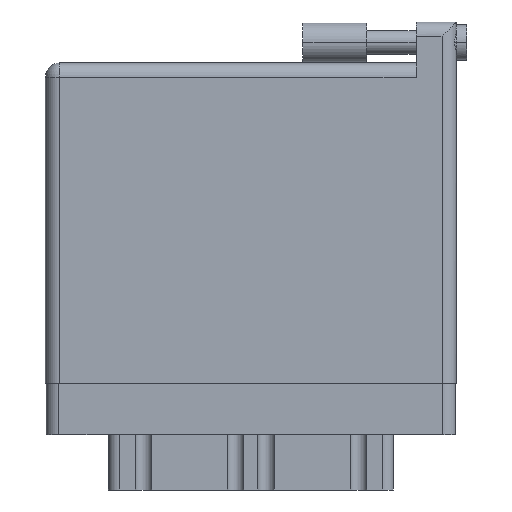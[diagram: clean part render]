
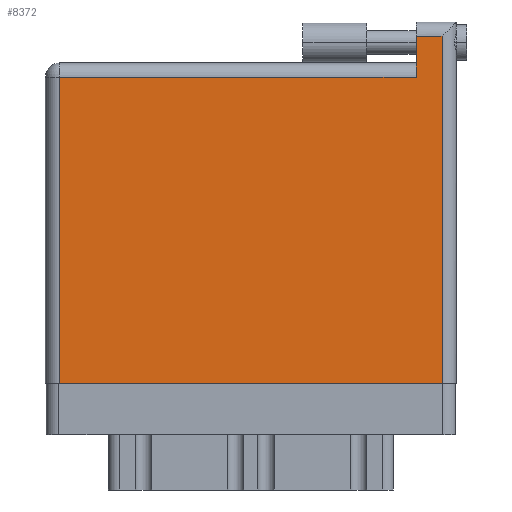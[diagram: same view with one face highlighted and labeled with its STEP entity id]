
A CAD part, front view. The second image highlights one B-rep face of the part: STEP entity #8372.
In plain terms, the highlighted face is planar.
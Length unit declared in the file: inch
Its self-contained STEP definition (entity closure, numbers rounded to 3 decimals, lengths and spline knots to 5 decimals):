
#135 = CARTESIAN_POINT ( 'NONE',  ( 0.07, 0., 0. ) ) ;
#1037 = CARTESIAN_POINT ( 'NONE',  ( 0., 1.696, 0. ) ) ;
#4168 = ORIENTED_EDGE ( 'NONE', *, *, #9324, .T. ) ;
#5502 = CARTESIAN_POINT ( 'NONE',  ( 0., 0., 0. ) ) ;
#5734 = DIRECTION ( 'NONE',  ( -1., 0., 0. ) ) ;
#6928 = LINE ( 'NONE', #24850, #19452 ) ;
#8372 = ADVANCED_FACE ( 'NONE', ( #17050 ), #26573, .F. ) ;
#8812 = CARTESIAN_POINT ( 'NONE',  ( 0.07, 1.496, 0. ) ) ;
#9324 = EDGE_CURVE ( 'NONE', #18946, #22883, #26620, .T. ) ;
#9838 = LINE ( 'NONE', #21716, #25200 ) ;
#10138 = VECTOR ( 'NONE', #36726, 39.37008 ) ;
#11650 = VECTOR ( 'NONE', #12889, 39.37008 ) ;
#12889 = DIRECTION ( 'NONE',  ( -1., 0., 0. ) ) ;
#13573 = CARTESIAN_POINT ( 'NONE',  ( 0.07, 0., 0. ) ) ;
#13674 = CARTESIAN_POINT ( 'NONE',  ( 1.938, 0., 0. ) ) ;
#14762 = EDGE_CURVE ( 'NONE', #27749, #20582, #28299, .T. ) ;
#15641 = CARTESIAN_POINT ( 'NONE',  ( 1.811, 1.496, 0. ) ) ;
#15845 = ORIENTED_EDGE ( 'NONE', *, *, #14762, .T. ) ;
#15882 = DIRECTION ( 'NONE',  ( 0., -1., 0. ) ) ;
#16023 = EDGE_CURVE ( 'NONE', #20582, #17755, #9838, .T. ) ;
#16431 = LINE ( 'NONE', #5502, #33387 ) ;
#16459 = CARTESIAN_POINT ( 'NONE',  ( 0., 1.496, 0. ) ) ;
#16797 = ORIENTED_EDGE ( 'NONE', *, *, #27980, .T. ) ;
#17050 = FACE_OUTER_BOUND ( 'NONE', #35633, .T. ) ;
#17755 = VERTEX_POINT ( 'NONE', #15641 ) ;
#18946 = VERTEX_POINT ( 'NONE', #8812 ) ;
#19452 = VECTOR ( 'NONE', #22445, 39.37008 ) ;
#19896 = AXIS2_PLACEMENT_3D ( 'NONE', #34985, #20336, #5734 ) ;
#20336 = DIRECTION ( 'NONE',  ( 0., 0., -1. ) ) ;
#20582 = VERTEX_POINT ( 'NONE', #32370 ) ;
#21716 = CARTESIAN_POINT ( 'NONE',  ( 1.811, 1.766, 0. ) ) ;
#22445 = DIRECTION ( 'NONE',  ( 0., 1., 0. ) ) ;
#22883 = VERTEX_POINT ( 'NONE', #13573 ) ;
#23702 = CARTESIAN_POINT ( 'NONE',  ( 1.938, 1.696, 0. ) ) ;
#23784 = ORIENTED_EDGE ( 'NONE', *, *, #36188, .T. ) ;
#24850 = CARTESIAN_POINT ( 'NONE',  ( 1.938, 1.766, 0. ) ) ;
#25200 = VECTOR ( 'NONE', #15882, 39.37008 ) ;
#26172 = EDGE_CURVE ( 'NONE', #17755, #18946, #31472, .T. ) ;
#26573 = PLANE ( 'NONE',  #19896 ) ;
#26620 = LINE ( 'NONE', #135, #34910 ) ;
#27749 = VERTEX_POINT ( 'NONE', #23702 ) ;
#27980 = EDGE_CURVE ( 'NONE', #28033, #27749, #6928, .T. ) ;
#28033 = VERTEX_POINT ( 'NONE', #13674 ) ;
#28299 = LINE ( 'NONE', #1037, #11650 ) ;
#29291 = DIRECTION ( 'NONE',  ( 1., 0., 0. ) ) ;
#31472 = LINE ( 'NONE', #16459, #10138 ) ;
#32370 = CARTESIAN_POINT ( 'NONE',  ( 1.811, 1.696, 0. ) ) ;
#33387 = VECTOR ( 'NONE', #29291, 39.37008 ) ;
#34910 = VECTOR ( 'NONE', #35611, 39.37008 ) ;
#34980 = ORIENTED_EDGE ( 'NONE', *, *, #26172, .T. ) ;
#34985 = CARTESIAN_POINT ( 'NONE',  ( 0., 1.566, 0. ) ) ;
#35611 = DIRECTION ( 'NONE',  ( 0., -1., 0. ) ) ;
#35633 = EDGE_LOOP ( 'NONE', ( #23784, #16797, #15845, #37068, #34980, #4168 ) ) ;
#36188 = EDGE_CURVE ( 'NONE', #22883, #28033, #16431, .T. ) ;
#36726 = DIRECTION ( 'NONE',  ( -1., 0., 0. ) ) ;
#37068 = ORIENTED_EDGE ( 'NONE', *, *, #16023, .T. ) ;
